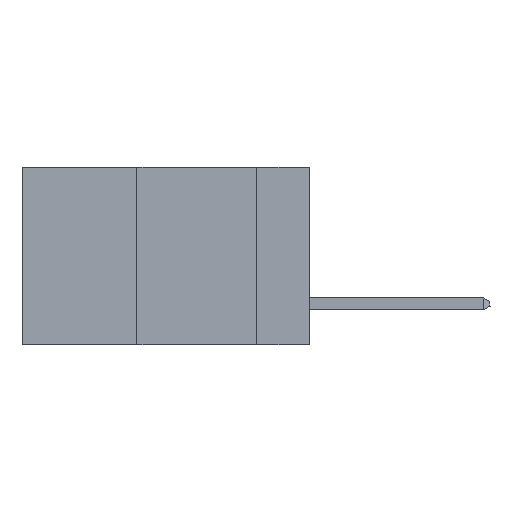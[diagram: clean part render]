
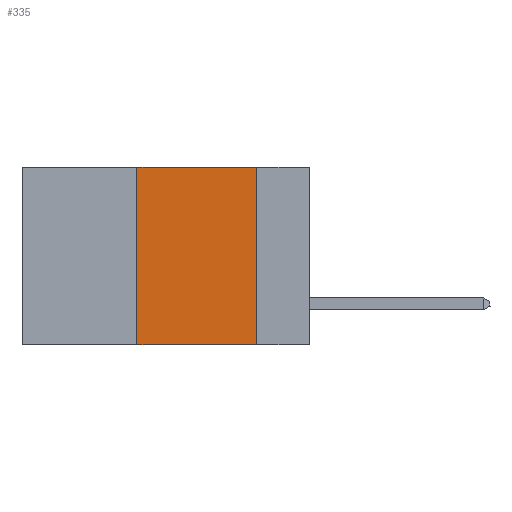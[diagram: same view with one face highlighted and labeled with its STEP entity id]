
A CAD part, left-side view. The second image highlights one B-rep face of the part: STEP entity #335.
In plain terms, the highlighted planar face has unit normal (-1, 0, 0).
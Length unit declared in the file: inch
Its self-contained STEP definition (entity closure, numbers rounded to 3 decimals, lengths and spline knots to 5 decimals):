
#265 = CARTESIAN_POINT ( 'NONE',  ( 0., 0.36, 0. ) ) ;
#335 = ADVANCED_FACE ( 'NONE', ( #4886 ), #2654, .F. ) ;
#727 = VERTEX_POINT ( 'NONE', #14897 ) ;
#733 = EDGE_CURVE ( 'NONE', #12632, #8105, #5789, .T. ) ;
#1284 = ORIENTED_EDGE ( 'NONE', *, *, #733, .F. ) ;
#1947 = DIRECTION ( 'NONE',  ( 0., -1., 0. ) ) ;
#2202 = VECTOR ( 'NONE', #10758, 39.37008 ) ;
#2654 = PLANE ( 'NONE',  #13734 ) ;
#3115 = DIRECTION ( 'NONE',  ( 0., 0., -1. ) ) ;
#3611 = VECTOR ( 'NONE', #1947, 39.37008 ) ;
#3823 = DIRECTION ( 'NONE',  ( 1., 0., 0. ) ) ;
#3827 = DIRECTION ( 'NONE',  ( 0., -1., 0. ) ) ;
#4041 = LINE ( 'NONE', #265, #2202 ) ;
#4118 = CARTESIAN_POINT ( 'NONE',  ( 0., 0.11, 0. ) ) ;
#4699 = EDGE_CURVE ( 'NONE', #7637, #727, #9147, .T. ) ;
#4886 = FACE_OUTER_BOUND ( 'NONE', #8813, .T. ) ;
#5789 = LINE ( 'NONE', #7881, #3611 ) ;
#6059 = CARTESIAN_POINT ( 'NONE',  ( 0., 0.6, -0.37 ) ) ;
#7637 = VERTEX_POINT ( 'NONE', #8995 ) ;
#7881 = CARTESIAN_POINT ( 'NONE',  ( 0., 0.6, 0. ) ) ;
#8105 = VERTEX_POINT ( 'NONE', #4118 ) ;
#8170 = EDGE_CURVE ( 'NONE', #8105, #727, #14669, .T. ) ;
#8813 = EDGE_LOOP ( 'NONE', ( #12039, #1284, #13450, #13233 ) ) ;
#8995 = CARTESIAN_POINT ( 'NONE',  ( 0., 0.36, -0.37 ) ) ;
#9147 = LINE ( 'NONE', #6059, #14603 ) ;
#9307 = CARTESIAN_POINT ( 'NONE',  ( 0., 0.11, 0. ) ) ;
#9491 = CARTESIAN_POINT ( 'NONE',  ( 0., 0.36, 0. ) ) ;
#10718 = DIRECTION ( 'NONE',  ( 0., 0., -1. ) ) ;
#10758 = DIRECTION ( 'NONE',  ( 0., 0., 1. ) ) ;
#10822 = CARTESIAN_POINT ( 'NONE',  ( 0., 0.6, 0. ) ) ;
#12039 = ORIENTED_EDGE ( 'NONE', *, *, #8170, .F. ) ;
#12079 = EDGE_CURVE ( 'NONE', #7637, #12632, #4041, .T. ) ;
#12632 = VERTEX_POINT ( 'NONE', #9491 ) ;
#13233 = ORIENTED_EDGE ( 'NONE', *, *, #4699, .T. ) ;
#13450 = ORIENTED_EDGE ( 'NONE', *, *, #12079, .F. ) ;
#13734 = AXIS2_PLACEMENT_3D ( 'NONE', #10822, #3823, #10718 ) ;
#14121 = VECTOR ( 'NONE', #3115, 39.37008 ) ;
#14603 = VECTOR ( 'NONE', #3827, 39.37008 ) ;
#14669 = LINE ( 'NONE', #9307, #14121 ) ;
#14897 = CARTESIAN_POINT ( 'NONE',  ( 0., 0.11, -0.37 ) ) ;
